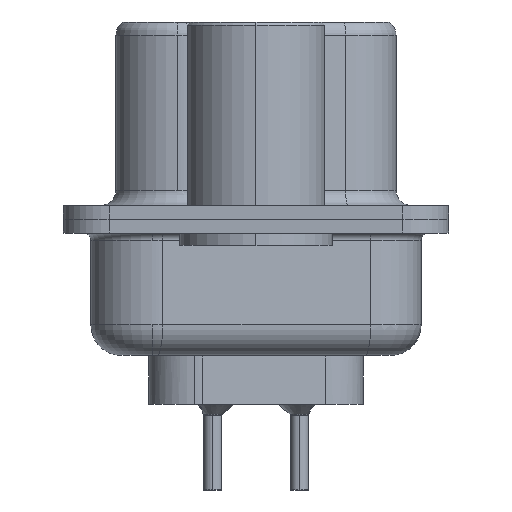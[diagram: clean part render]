
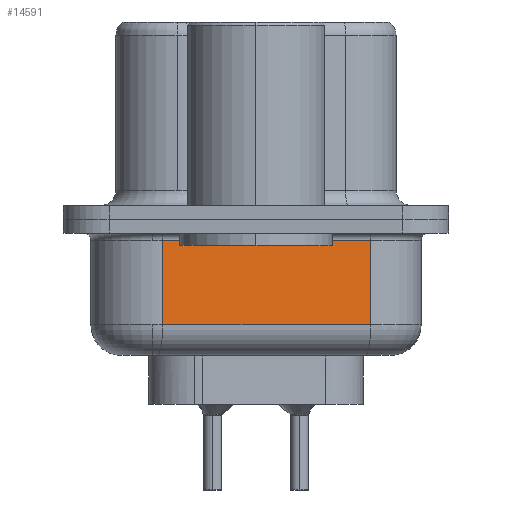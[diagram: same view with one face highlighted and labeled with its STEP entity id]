
A CAD part, left-side view. The second image highlights one B-rep face of the part: STEP entity #14591.
In plain terms, the highlighted planar face has unit normal (-0.985, -0.174, 0).
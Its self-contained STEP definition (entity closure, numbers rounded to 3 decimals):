
#648 = EDGE_CURVE ( 'NONE', #8401, #7673, #6643, .T. ) ;
#1250 = DIRECTION ( 'NONE',  ( 0.985, 0.174, 0. ) ) ;
#1337 = CARTESIAN_POINT ( 'NONE',  ( 2.875, 3.053, -0.7 ) ) ;
#1902 = CARTESIAN_POINT ( 'NONE',  ( 4.074, -3.747, -3.45 ) ) ;
#2677 = ORIENTED_EDGE ( 'NONE', *, *, #648, .T. ) ;
#3113 = VECTOR ( 'NONE', #10800, 1000. ) ;
#3320 = LINE ( 'NONE', #5782, #18727 ) ;
#4246 = VECTOR ( 'NONE', #11017, 1000. ) ;
#5164 = EDGE_CURVE ( 'NONE', #6040, #16986, #8213, .T. ) ;
#5782 = CARTESIAN_POINT ( 'NONE',  ( 2.875, 3.053, -4.45 ) ) ;
#5915 = AXIS2_PLACEMENT_3D ( 'NONE', #14660, #1250, #11746 ) ;
#6040 = VERTEX_POINT ( 'NONE', #13159 ) ;
#6643 = LINE ( 'NONE', #6954, #14587 ) ;
#6954 = CARTESIAN_POINT ( 'NONE',  ( 2.875, 3.053, -0.7 ) ) ;
#7237 = PLANE ( 'NONE',  #5915 ) ;
#7458 = DIRECTION ( 'NONE',  ( -0.174, 0.985, 0. ) ) ;
#7666 = ORIENTED_EDGE ( 'NONE', *, *, #5164, .T. ) ;
#7673 = VERTEX_POINT ( 'NONE', #1337 ) ;
#8213 = LINE ( 'NONE', #16940, #4246 ) ;
#8401 = VERTEX_POINT ( 'NONE', #18720 ) ;
#9047 = FACE_OUTER_BOUND ( 'NONE', #19149, .T. ) ;
#10307 = DIRECTION ( 'NONE',  ( 0., 0., 1. ) ) ;
#10649 = EDGE_CURVE ( 'NONE', #6040, #7673, #3320, .T. ) ;
#10800 = DIRECTION ( 'NONE',  ( 0., 0., 1. ) ) ;
#11017 = DIRECTION ( 'NONE',  ( 0.174, -0.985, 0. ) ) ;
#11746 = DIRECTION ( 'NONE',  ( -0.174, 0.985, 0. ) ) ;
#12016 = LINE ( 'NONE', #13807, #3113 ) ;
#13000 = ORIENTED_EDGE ( 'NONE', *, *, #10649, .F. ) ;
#13159 = CARTESIAN_POINT ( 'NONE',  ( 2.875, 3.053, -3.45 ) ) ;
#13807 = CARTESIAN_POINT ( 'NONE',  ( 4.074, -3.747, -4.45 ) ) ;
#14587 = VECTOR ( 'NONE', #7458, 1000. ) ;
#14591 = ADVANCED_FACE ( 'NONE', ( #9047 ), #7237, .F. ) ;
#14660 = CARTESIAN_POINT ( 'NONE',  ( 2.875, 3.053, -4.45 ) ) ;
#16940 = CARTESIAN_POINT ( 'NONE',  ( 2.875, 3.053, -3.45 ) ) ;
#16955 = EDGE_CURVE ( 'NONE', #16986, #8401, #12016, .T. ) ;
#16986 = VERTEX_POINT ( 'NONE', #1902 ) ;
#18720 = CARTESIAN_POINT ( 'NONE',  ( 4.074, -3.747, -0.7 ) ) ;
#18727 = VECTOR ( 'NONE', #10307, 1000. ) ;
#18870 = ORIENTED_EDGE ( 'NONE', *, *, #16955, .T. ) ;
#19149 = EDGE_LOOP ( 'NONE', ( #13000, #7666, #18870, #2677 ) ) ;
